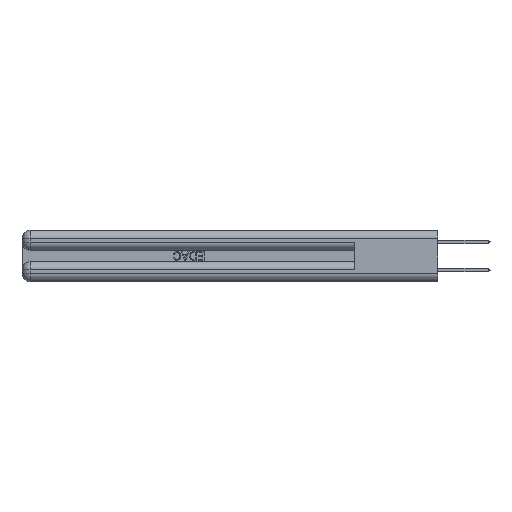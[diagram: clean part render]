
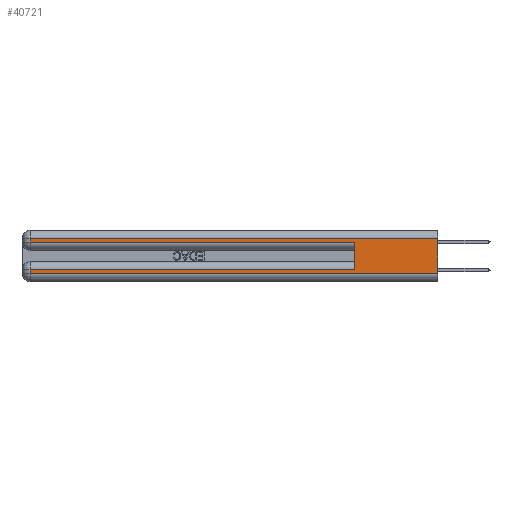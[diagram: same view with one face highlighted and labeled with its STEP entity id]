
A CAD part, left-side view. The second image highlights one B-rep face of the part: STEP entity #40721.
In plain terms, the highlighted planar face has unit normal (-1, 0, 0).
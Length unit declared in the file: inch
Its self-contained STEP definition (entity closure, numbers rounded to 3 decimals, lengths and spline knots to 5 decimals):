
#860 = DIRECTION ( 'NONE',  ( 0., 0., -1. ) ) ;
#1900 = DIRECTION ( 'NONE',  ( 0., 0., -1. ) ) ;
#3337 = VERTEX_POINT ( 'NONE', #7110 ) ;
#3691 = EDGE_CURVE ( 'NONE', #32399, #33019, #9225, .T. ) ;
#4428 = VECTOR ( 'NONE', #34914, 39.37008 ) ;
#4883 = EDGE_CURVE ( 'NONE', #22185, #3337, #23070, .T. ) ;
#5079 = CARTESIAN_POINT ( 'NONE',  ( 0., 0.6, 0.285 ) ) ;
#6167 = LINE ( 'NONE', #33800, #13907 ) ;
#7110 = CARTESIAN_POINT ( 'NONE',  ( 0., 2.94, 0.31 ) ) ;
#7745 = ORIENTED_EDGE ( 'NONE', *, *, #11197, .F. ) ;
#9074 = PLANE ( 'NONE',  #9608 ) ;
#9225 = LINE ( 'NONE', #16921, #34532 ) ;
#9252 = CARTESIAN_POINT ( 'NONE',  ( 0., 0.6, 0.085 ) ) ;
#9599 = ORIENTED_EDGE ( 'NONE', *, *, #37748, .T. ) ;
#9608 = AXIS2_PLACEMENT_3D ( 'NONE', #15687, #38782, #19036 ) ;
#10034 = DIRECTION ( 'NONE',  ( 0., 1., 0. ) ) ;
#10571 = CARTESIAN_POINT ( 'NONE',  ( 0., 2.94, 0.06 ) ) ;
#10905 = DIRECTION ( 'NONE',  ( 0., 0., -1. ) ) ;
#10964 = VERTEX_POINT ( 'NONE', #26767 ) ;
#11197 = EDGE_CURVE ( 'NONE', #32399, #41643, #25732, .T. ) ;
#13224 = ORIENTED_EDGE ( 'NONE', *, *, #4883, .T. ) ;
#13907 = VECTOR ( 'NONE', #860, 39.37008 ) ;
#15120 = EDGE_CURVE ( 'NONE', #22185, #39824, #19218, .T. ) ;
#15687 = CARTESIAN_POINT ( 'NONE',  ( 0., 0., 0.37 ) ) ;
#15842 = LINE ( 'NONE', #21717, #39089 ) ;
#16209 = ORIENTED_EDGE ( 'NONE', *, *, #19478, .T. ) ;
#16921 = CARTESIAN_POINT ( 'NONE',  ( 0., 0., 0.085 ) ) ;
#18161 = ORIENTED_EDGE ( 'NONE', *, *, #26446, .T. ) ;
#18461 = CARTESIAN_POINT ( 'NONE',  ( 0., 0., 0.06 ) ) ;
#18690 = DIRECTION ( 'NONE',  ( 0., -1., 0. ) ) ;
#19036 = DIRECTION ( 'NONE',  ( 0., 0., -1. ) ) ;
#19103 = EDGE_LOOP ( 'NONE', ( #23404, #13224, #18161, #39096, #7745, #21735, #9599, #16209 ) ) ;
#19218 = LINE ( 'NONE', #27383, #36777 ) ;
#19478 = EDGE_CURVE ( 'NONE', #24352, #39824, #30771, .T. ) ;
#20243 = DIRECTION ( 'NONE',  ( 0., 1., 0. ) ) ;
#21618 = CARTESIAN_POINT ( 'NONE',  ( 0., 0., 0.31 ) ) ;
#21717 = CARTESIAN_POINT ( 'NONE',  ( 0., 2.94, 0.37 ) ) ;
#21735 = ORIENTED_EDGE ( 'NONE', *, *, #3691, .T. ) ;
#22185 = VERTEX_POINT ( 'NONE', #21618 ) ;
#23070 = LINE ( 'NONE', #29828, #31810 ) ;
#23404 = ORIENTED_EDGE ( 'NONE', *, *, #15120, .F. ) ;
#24352 = VERTEX_POINT ( 'NONE', #10571 ) ;
#24721 = CARTESIAN_POINT ( 'NONE',  ( 0., 0., 0.06 ) ) ;
#25501 = CARTESIAN_POINT ( 'NONE',  ( 0., 2.94, 0.085 ) ) ;
#25732 = LINE ( 'NONE', #37731, #33486 ) ;
#26440 = VECTOR ( 'NONE', #18690, 39.37008 ) ;
#26446 = EDGE_CURVE ( 'NONE', #3337, #10964, #15842, .T. ) ;
#26767 = CARTESIAN_POINT ( 'NONE',  ( 0., 2.94, 0.285 ) ) ;
#27383 = CARTESIAN_POINT ( 'NONE',  ( 0., 0., 0.37 ) ) ;
#27483 = LINE ( 'NONE', #35143, #26440 ) ;
#28019 = FACE_OUTER_BOUND ( 'NONE', #19103, .T. ) ;
#29828 = CARTESIAN_POINT ( 'NONE',  ( 0., 0., 0.31 ) ) ;
#30771 = LINE ( 'NONE', #18461, #4428 ) ;
#31683 = EDGE_CURVE ( 'NONE', #10964, #41643, #27483, .T. ) ;
#31810 = VECTOR ( 'NONE', #10034, 39.37008 ) ;
#32399 = VERTEX_POINT ( 'NONE', #9252 ) ;
#33019 = VERTEX_POINT ( 'NONE', #25501 ) ;
#33486 = VECTOR ( 'NONE', #41025, 39.37008 ) ;
#33800 = CARTESIAN_POINT ( 'NONE',  ( 0., 2.94, 0.37 ) ) ;
#34532 = VECTOR ( 'NONE', #20243, 39.37008 ) ;
#34914 = DIRECTION ( 'NONE',  ( 0., -1., 0. ) ) ;
#35143 = CARTESIAN_POINT ( 'NONE',  ( 0., 0., 0.285 ) ) ;
#36777 = VECTOR ( 'NONE', #10905, 39.37008 ) ;
#37731 = CARTESIAN_POINT ( 'NONE',  ( 0., 0.6, 0.145 ) ) ;
#37748 = EDGE_CURVE ( 'NONE', #33019, #24352, #6167, .T. ) ;
#38782 = DIRECTION ( 'NONE',  ( 1., 0., 0. ) ) ;
#39089 = VECTOR ( 'NONE', #1900, 39.37008 ) ;
#39096 = ORIENTED_EDGE ( 'NONE', *, *, #31683, .T. ) ;
#39824 = VERTEX_POINT ( 'NONE', #24721 ) ;
#40721 = ADVANCED_FACE ( 'NONE', ( #28019 ), #9074, .F. ) ;
#41025 = DIRECTION ( 'NONE',  ( 0., 0., 1. ) ) ;
#41643 = VERTEX_POINT ( 'NONE', #5079 ) ;
